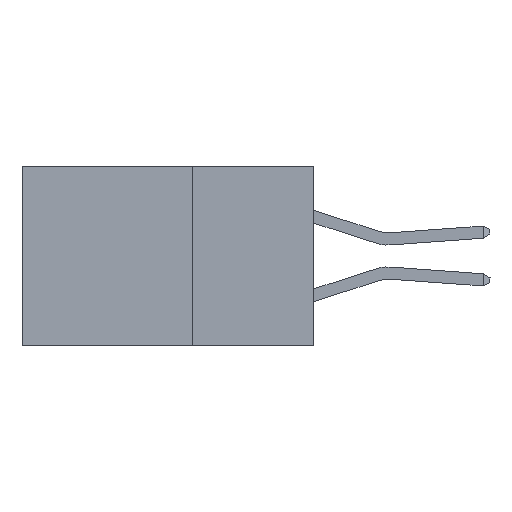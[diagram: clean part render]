
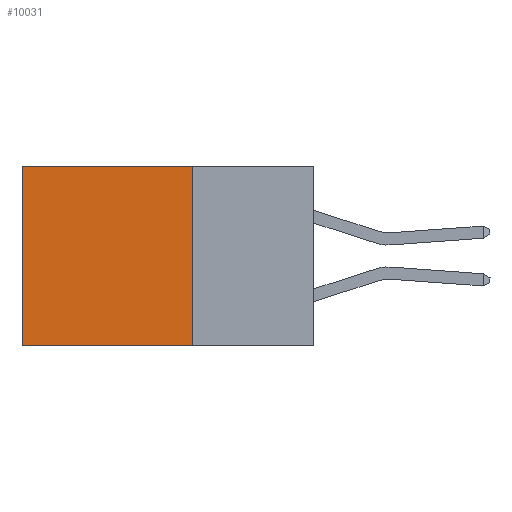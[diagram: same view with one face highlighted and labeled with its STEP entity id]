
A CAD part, left-side view. The second image highlights one B-rep face of the part: STEP entity #10031.
In plain terms, the highlighted planar face has unit normal (-1, 0, 0).
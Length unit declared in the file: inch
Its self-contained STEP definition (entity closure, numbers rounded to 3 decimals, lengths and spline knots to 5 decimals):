
#6 = VECTOR ( 'NONE', #7873, 39.37008 ) ;
#1381 = ORIENTED_EDGE ( 'NONE', *, *, #4208, .T. ) ;
#1389 = PLANE ( 'NONE',  #3213 ) ;
#1474 = DIRECTION ( 'NONE',  ( 0., 0., -1. ) ) ;
#1524 = CARTESIAN_POINT ( 'NONE',  ( 0.2875, 0.25, -0.37 ) ) ;
#1927 = VECTOR ( 'NONE', #9930, 39.37008 ) ;
#2555 = CARTESIAN_POINT ( 'NONE',  ( 0.2875, 0.25, 0. ) ) ;
#2664 = VERTEX_POINT ( 'NONE', #8348 ) ;
#3011 = DIRECTION ( 'NONE',  ( 1., 0., 0. ) ) ;
#3213 = AXIS2_PLACEMENT_3D ( 'NONE', #3928, #3011, #1474 ) ;
#3362 = ORIENTED_EDGE ( 'NONE', *, *, #7887, .F. ) ;
#3928 = CARTESIAN_POINT ( 'NONE',  ( 0.2875, 0.25, 0. ) ) ;
#3952 = EDGE_LOOP ( 'NONE', ( #1381, #6041, #3362, #5029 ) ) ;
#4208 = EDGE_CURVE ( 'NONE', #4832, #2664, #8976, .T. ) ;
#4267 = DIRECTION ( 'NONE',  ( 0., 0., -1. ) ) ;
#4494 = LINE ( 'NONE', #8839, #4767 ) ;
#4767 = VECTOR ( 'NONE', #9684, 39.37008 ) ;
#4803 = FACE_OUTER_BOUND ( 'NONE', #3952, .T. ) ;
#4832 = VERTEX_POINT ( 'NONE', #10570 ) ;
#4890 = CARTESIAN_POINT ( 'NONE',  ( 0.2875, 0.25, 0. ) ) ;
#5029 = ORIENTED_EDGE ( 'NONE', *, *, #9627, .T. ) ;
#5285 = LINE ( 'NONE', #10837, #1927 ) ;
#6041 = ORIENTED_EDGE ( 'NONE', *, *, #11239, .F. ) ;
#6656 = LINE ( 'NONE', #2555, #6 ) ;
#7873 = DIRECTION ( 'NONE',  ( 0., 1., 0. ) ) ;
#7887 = EDGE_CURVE ( 'NONE', #8609, #9700, #5285, .T. ) ;
#8348 = CARTESIAN_POINT ( 'NONE',  ( 0.2875, 0.6, -0.37 ) ) ;
#8609 = VERTEX_POINT ( 'NONE', #4890 ) ;
#8666 = CARTESIAN_POINT ( 'NONE',  ( 0.2875, 0.6, 0. ) ) ;
#8839 = CARTESIAN_POINT ( 'NONE',  ( 0.2875, 0.25, -0.37 ) ) ;
#8976 = LINE ( 'NONE', #8666, #11063 ) ;
#9627 = EDGE_CURVE ( 'NONE', #8609, #4832, #6656, .T. ) ;
#9684 = DIRECTION ( 'NONE',  ( 0., 1., 0. ) ) ;
#9700 = VERTEX_POINT ( 'NONE', #1524 ) ;
#9930 = DIRECTION ( 'NONE',  ( 0., 0., -1. ) ) ;
#10031 = ADVANCED_FACE ( 'NONE', ( #4803 ), #1389, .F. ) ;
#10570 = CARTESIAN_POINT ( 'NONE',  ( 0.2875, 0.6, 0. ) ) ;
#10837 = CARTESIAN_POINT ( 'NONE',  ( 0.2875, 0.25, 0. ) ) ;
#11063 = VECTOR ( 'NONE', #4267, 39.37008 ) ;
#11239 = EDGE_CURVE ( 'NONE', #9700, #2664, #4494, .T. ) ;
